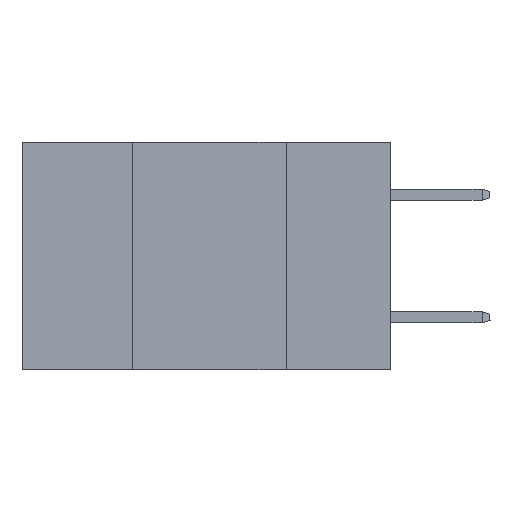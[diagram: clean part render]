
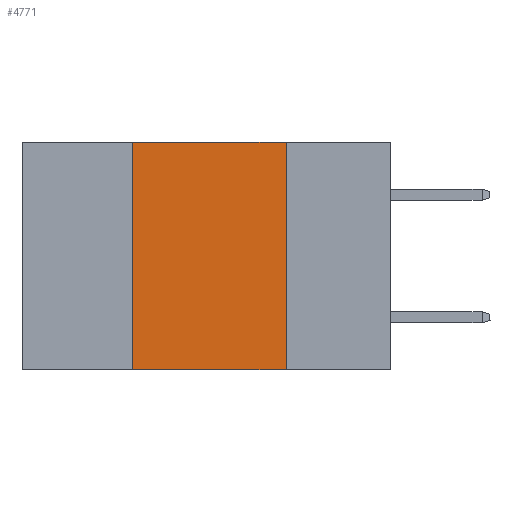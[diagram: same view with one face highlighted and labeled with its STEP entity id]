
A CAD part, left-side view. The second image highlights one B-rep face of the part: STEP entity #4771.
In plain terms, the highlighted planar face has unit normal (-1, 0, 0).
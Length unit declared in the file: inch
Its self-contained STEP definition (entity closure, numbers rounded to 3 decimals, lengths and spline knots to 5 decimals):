
#423 = DIRECTION ( 'NONE',  ( 0., 0., -1. ) ) ;
#1635 = AXIS2_PLACEMENT_3D ( 'NONE', #16818, #6095, #3900 ) ;
#2839 = VECTOR ( 'NONE', #10299, 39.37008 ) ;
#3900 = DIRECTION ( 'NONE',  ( 0., 0., -1. ) ) ;
#4771 = ADVANCED_FACE ( 'NONE', ( #8270 ), #5952, .F. ) ;
#5952 = PLANE ( 'NONE',  #1635 ) ;
#6038 = VERTEX_POINT ( 'NONE', #12572 ) ;
#6095 = DIRECTION ( 'NONE',  ( 1., 0., 0. ) ) ;
#6254 = EDGE_CURVE ( 'NONE', #6038, #11765, #19518, .T. ) ;
#6276 = EDGE_LOOP ( 'NONE', ( #8542, #25944, #13994, #23976 ) ) ;
#6722 = CARTESIAN_POINT ( 'NONE',  ( 0., 0.6, 0. ) ) ;
#7703 = VERTEX_POINT ( 'NONE', #15288 ) ;
#8270 = FACE_OUTER_BOUND ( 'NONE', #6276, .T. ) ;
#8542 = ORIENTED_EDGE ( 'NONE', *, *, #9314, .F. ) ;
#9314 = EDGE_CURVE ( 'NONE', #11765, #7703, #14987, .T. ) ;
#10299 = DIRECTION ( 'NONE',  ( 0., -1., 0. ) ) ;
#11090 = VECTOR ( 'NONE', #11095, 39.37008 ) ;
#11095 = DIRECTION ( 'NONE',  ( 0., 0., 1. ) ) ;
#11524 = VECTOR ( 'NONE', #17312, 39.37008 ) ;
#11765 = VERTEX_POINT ( 'NONE', #14060 ) ;
#11778 = CARTESIAN_POINT ( 'NONE',  ( 0., 0.42, -0.37 ) ) ;
#12572 = CARTESIAN_POINT ( 'NONE',  ( 0., 0.42, 0. ) ) ;
#13994 = ORIENTED_EDGE ( 'NONE', *, *, #21028, .F. ) ;
#14060 = CARTESIAN_POINT ( 'NONE',  ( 0., 0.17, 0. ) ) ;
#14987 = LINE ( 'NONE', #16921, #18015 ) ;
#15288 = CARTESIAN_POINT ( 'NONE',  ( 0., 0.17, -0.37 ) ) ;
#16818 = CARTESIAN_POINT ( 'NONE',  ( 0., 0.6, 0. ) ) ;
#16921 = CARTESIAN_POINT ( 'NONE',  ( 0., 0.17, 0. ) ) ;
#17312 = DIRECTION ( 'NONE',  ( 0., -1., 0. ) ) ;
#18015 = VECTOR ( 'NONE', #423, 39.37008 ) ;
#18412 = CARTESIAN_POINT ( 'NONE',  ( 0., 0.6, -0.37 ) ) ;
#19518 = LINE ( 'NONE', #6722, #11524 ) ;
#21028 = EDGE_CURVE ( 'NONE', #23912, #6038, #21550, .T. ) ;
#21550 = LINE ( 'NONE', #25372, #11090 ) ;
#22252 = EDGE_CURVE ( 'NONE', #23912, #7703, #26895, .T. ) ;
#23912 = VERTEX_POINT ( 'NONE', #11778 ) ;
#23976 = ORIENTED_EDGE ( 'NONE', *, *, #22252, .T. ) ;
#25372 = CARTESIAN_POINT ( 'NONE',  ( 0., 0.42, 0. ) ) ;
#25944 = ORIENTED_EDGE ( 'NONE', *, *, #6254, .F. ) ;
#26895 = LINE ( 'NONE', #18412, #2839 ) ;
